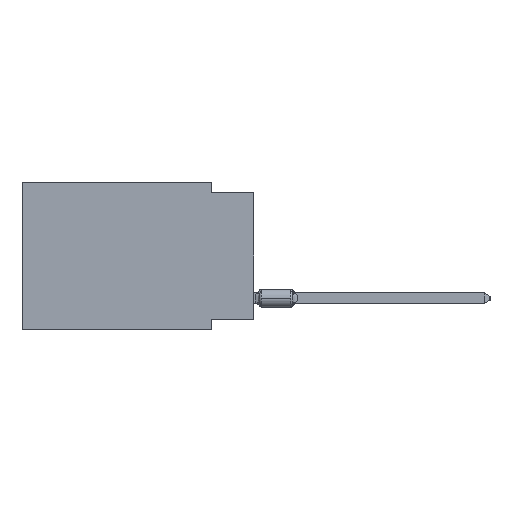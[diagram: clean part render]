
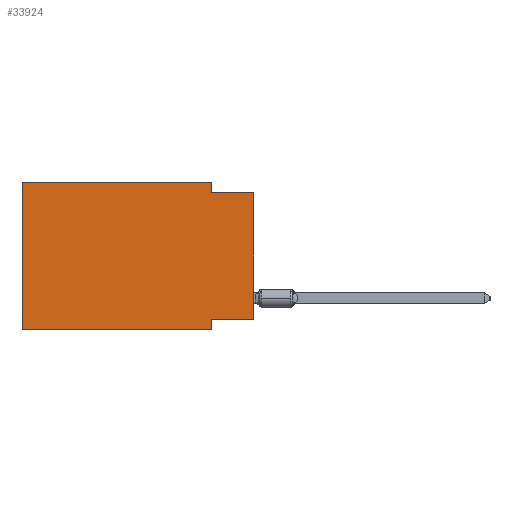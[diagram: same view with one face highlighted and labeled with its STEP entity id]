
A CAD part, left-side view. The second image highlights one B-rep face of the part: STEP entity #33924.
In plain terms, the highlighted planar face has unit normal (-1, 0, 0).
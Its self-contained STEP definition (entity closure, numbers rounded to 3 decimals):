
#420 = CARTESIAN_POINT ( 'NONE',  ( 0., 2.54, -8.89 ) ) ;
#1754 = CARTESIAN_POINT ( 'NONE',  ( 0., 0., -8.255 ) ) ;
#1851 = LINE ( 'NONE', #38890, #42374 ) ;
#1881 = ORIENTED_EDGE ( 'NONE', *, *, #34332, .F. ) ;
#2925 = DIRECTION ( 'NONE',  ( 0., 1., 0. ) ) ;
#2990 = DIRECTION ( 'NONE',  ( 0., 0., -1. ) ) ;
#3614 = CARTESIAN_POINT ( 'NONE',  ( 0., 2.54, -8.255 ) ) ;
#4114 = VERTEX_POINT ( 'NONE', #17794 ) ;
#5304 = CARTESIAN_POINT ( 'NONE',  ( 0., 13.97, -8.89 ) ) ;
#6985 = ORIENTED_EDGE ( 'NONE', *, *, #34726, .F. ) ;
#7498 = LINE ( 'NONE', #40574, #32274 ) ;
#8083 = VERTEX_POINT ( 'NONE', #5304 ) ;
#9559 = DIRECTION ( 'NONE',  ( 0., -1., 0. ) ) ;
#9857 = VERTEX_POINT ( 'NONE', #420 ) ;
#10318 = FACE_OUTER_BOUND ( 'NONE', #19718, .T. ) ;
#11585 = LINE ( 'NONE', #41343, #39381 ) ;
#11897 = VECTOR ( 'NONE', #14812, 1000. ) ;
#12972 = DIRECTION ( 'NONE',  ( 0., 0., -1. ) ) ;
#13352 = ORIENTED_EDGE ( 'NONE', *, *, #39934, .F. ) ;
#13365 = CARTESIAN_POINT ( 'NONE',  ( 0., 0., -0.635 ) ) ;
#14414 = VECTOR ( 'NONE', #43288, 1000. ) ;
#14812 = DIRECTION ( 'NONE',  ( 0., -1., 0. ) ) ;
#16111 = LINE ( 'NONE', #29546, #35137 ) ;
#16488 = CARTESIAN_POINT ( 'NONE',  ( 0., 13.97, 0. ) ) ;
#17341 = EDGE_CURVE ( 'NONE', #26062, #29891, #1851, .T. ) ;
#17794 = CARTESIAN_POINT ( 'NONE',  ( 0., 13.97, 0. ) ) ;
#18830 = DIRECTION ( 'NONE',  ( 0., 0., -1. ) ) ;
#19341 = VERTEX_POINT ( 'NONE', #24450 ) ;
#19718 = EDGE_LOOP ( 'NONE', ( #23697, #26548, #1881, #6985, #13352, #23810, #30410, #41598 ) ) ;
#20276 = AXIS2_PLACEMENT_3D ( 'NONE', #16488, #23740, #12972 ) ;
#22578 = LINE ( 'NONE', #29631, #14414 ) ;
#23697 = ORIENTED_EDGE ( 'NONE', *, *, #36010, .T. ) ;
#23740 = DIRECTION ( 'NONE',  ( 1., 0., 0. ) ) ;
#23810 = ORIENTED_EDGE ( 'NONE', *, *, #28475, .T. ) ;
#24017 = DIRECTION ( 'NONE',  ( 0., 0., 1. ) ) ;
#24450 = CARTESIAN_POINT ( 'NONE',  ( 0., 2.54, 0. ) ) ;
#25163 = LINE ( 'NONE', #28464, #11897 ) ;
#26062 = VERTEX_POINT ( 'NONE', #1754 ) ;
#26548 = ORIENTED_EDGE ( 'NONE', *, *, #35850, .F. ) ;
#26675 = VECTOR ( 'NONE', #9559, 1000. ) ;
#26723 = CARTESIAN_POINT ( 'NONE',  ( 0., 13.97, 0. ) ) ;
#28464 = CARTESIAN_POINT ( 'NONE',  ( 0., 0., -0.635 ) ) ;
#28475 = EDGE_CURVE ( 'NONE', #8083, #9857, #22578, .T. ) ;
#29546 = CARTESIAN_POINT ( 'NONE',  ( 0., 0., 0. ) ) ;
#29631 = CARTESIAN_POINT ( 'NONE',  ( 0., 13.97, -8.89 ) ) ;
#29891 = VERTEX_POINT ( 'NONE', #3614 ) ;
#30313 = CARTESIAN_POINT ( 'NONE',  ( 0., 2.54, 0. ) ) ;
#30410 = ORIENTED_EDGE ( 'NONE', *, *, #40892, .F. ) ;
#32274 = VECTOR ( 'NONE', #24017, 1000. ) ;
#33924 = ADVANCED_FACE ( 'NONE', ( #10318 ), #36780, .F. ) ;
#34332 = EDGE_CURVE ( 'NONE', #19341, #43605, #39813, .T. ) ;
#34726 = EDGE_CURVE ( 'NONE', #4114, #19341, #43266, .T. ) ;
#35137 = VECTOR ( 'NONE', #35740, 1000. ) ;
#35740 = DIRECTION ( 'NONE',  ( 0., 0., 1. ) ) ;
#35850 = EDGE_CURVE ( 'NONE', #43605, #40775, #25163, .T. ) ;
#36010 = EDGE_CURVE ( 'NONE', #26062, #40775, #16111, .T. ) ;
#36780 = PLANE ( 'NONE',  #20276 ) ;
#37239 = VECTOR ( 'NONE', #2990, 1000. ) ;
#38890 = CARTESIAN_POINT ( 'NONE',  ( 0., 0., -8.255 ) ) ;
#39177 = CARTESIAN_POINT ( 'NONE',  ( 0., 2.54, -0.635 ) ) ;
#39381 = VECTOR ( 'NONE', #18830, 1000. ) ;
#39813 = LINE ( 'NONE', #30313, #37239 ) ;
#39934 = EDGE_CURVE ( 'NONE', #8083, #4114, #7498, .T. ) ;
#40574 = CARTESIAN_POINT ( 'NONE',  ( 0., 13.97, 0. ) ) ;
#40775 = VERTEX_POINT ( 'NONE', #13365 ) ;
#40892 = EDGE_CURVE ( 'NONE', #29891, #9857, #11585, .T. ) ;
#41343 = CARTESIAN_POINT ( 'NONE',  ( 0., 2.54, -8.89 ) ) ;
#41598 = ORIENTED_EDGE ( 'NONE', *, *, #17341, .F. ) ;
#42374 = VECTOR ( 'NONE', #2925, 1000. ) ;
#43266 = LINE ( 'NONE', #26723, #26675 ) ;
#43288 = DIRECTION ( 'NONE',  ( 0., -1., 0. ) ) ;
#43605 = VERTEX_POINT ( 'NONE', #39177 ) ;
